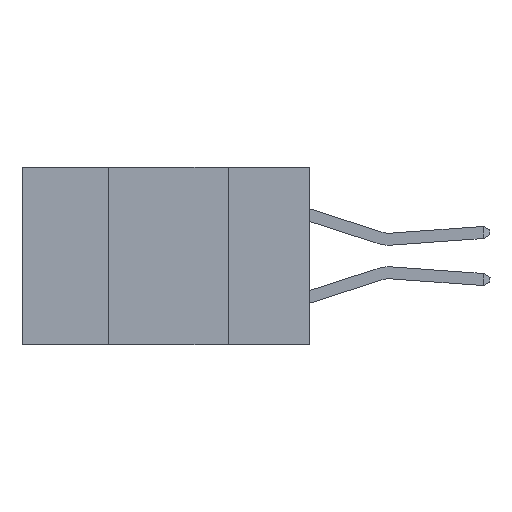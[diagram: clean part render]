
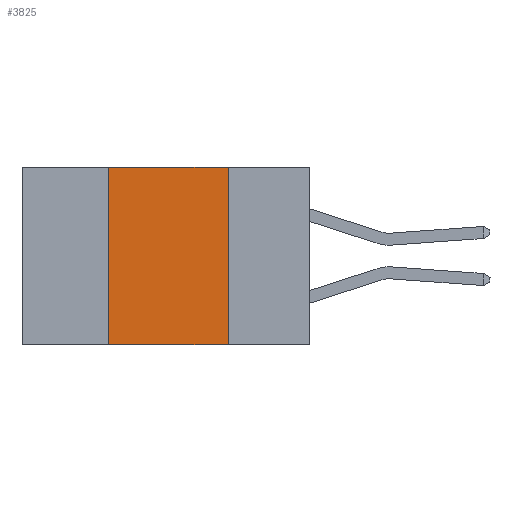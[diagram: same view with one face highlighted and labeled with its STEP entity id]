
A CAD part, left-side view. The second image highlights one B-rep face of the part: STEP entity #3825.
In plain terms, the highlighted planar face has unit normal (-1, 0, 0).
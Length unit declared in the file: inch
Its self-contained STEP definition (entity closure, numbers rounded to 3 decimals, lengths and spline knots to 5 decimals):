
#227 = VERTEX_POINT ( 'NONE', #5763 ) ;
#314 = FACE_OUTER_BOUND ( 'NONE', #3190, .T. ) ;
#378 = EDGE_CURVE ( 'NONE', #7599, #467, #10037, .T. ) ;
#467 = VERTEX_POINT ( 'NONE', #3789 ) ;
#687 = EDGE_CURVE ( 'NONE', #467, #6701, #10279, .T. ) ;
#803 = CARTESIAN_POINT ( 'NONE',  ( 0., 0.42, 0. ) ) ;
#828 = DIRECTION ( 'NONE',  ( 0., 0., -1. ) ) ;
#1116 = CARTESIAN_POINT ( 'NONE',  ( 0., 0.6, 0. ) ) ;
#1227 = DIRECTION ( 'NONE',  ( 0., -1., 0. ) ) ;
#2012 = LINE ( 'NONE', #5984, #7823 ) ;
#2166 = ORIENTED_EDGE ( 'NONE', *, *, #687, .F. ) ;
#2491 = ORIENTED_EDGE ( 'NONE', *, *, #4843, .F. ) ;
#2935 = LINE ( 'NONE', #3427, #6877 ) ;
#3190 = EDGE_LOOP ( 'NONE', ( #2166, #10221, #2491, #9879 ) ) ;
#3427 = CARTESIAN_POINT ( 'NONE',  ( 0., 0.42, -0.37 ) ) ;
#3789 = CARTESIAN_POINT ( 'NONE',  ( 0., 0.17, 0. ) ) ;
#3825 = ADVANCED_FACE ( 'NONE', ( #314 ), #6488, .F. ) ;
#4818 = CARTESIAN_POINT ( 'NONE',  ( 0., 0.6, 0. ) ) ;
#4843 = EDGE_CURVE ( 'NONE', #227, #7599, #2935, .T. ) ;
#4845 = CARTESIAN_POINT ( 'NONE',  ( 0., 0.17, -0.37 ) ) ;
#4871 = DIRECTION ( 'NONE',  ( 0., 0., -1. ) ) ;
#5763 = CARTESIAN_POINT ( 'NONE',  ( 0., 0.42, -0.37 ) ) ;
#5890 = DIRECTION ( 'NONE',  ( 0., -1., 0. ) ) ;
#5984 = CARTESIAN_POINT ( 'NONE',  ( 0., 0.6, -0.37 ) ) ;
#6488 = PLANE ( 'NONE',  #9583 ) ;
#6528 = DIRECTION ( 'NONE',  ( 0., 0., 1. ) ) ;
#6701 = VERTEX_POINT ( 'NONE', #4845 ) ;
#6877 = VECTOR ( 'NONE', #6528, 39.37008 ) ;
#7350 = EDGE_CURVE ( 'NONE', #227, #6701, #2012, .T. ) ;
#7412 = VECTOR ( 'NONE', #4871, 39.37008 ) ;
#7599 = VERTEX_POINT ( 'NONE', #803 ) ;
#7823 = VECTOR ( 'NONE', #1227, 39.37008 ) ;
#9279 = VECTOR ( 'NONE', #5890, 39.37008 ) ;
#9564 = CARTESIAN_POINT ( 'NONE',  ( 0., 0.17, -0.37 ) ) ;
#9573 = DIRECTION ( 'NONE',  ( 1., 0., 0. ) ) ;
#9583 = AXIS2_PLACEMENT_3D ( 'NONE', #4818, #9573, #828 ) ;
#9879 = ORIENTED_EDGE ( 'NONE', *, *, #7350, .T. ) ;
#10037 = LINE ( 'NONE', #1116, #9279 ) ;
#10221 = ORIENTED_EDGE ( 'NONE', *, *, #378, .F. ) ;
#10279 = LINE ( 'NONE', #9564, #7412 ) ;
